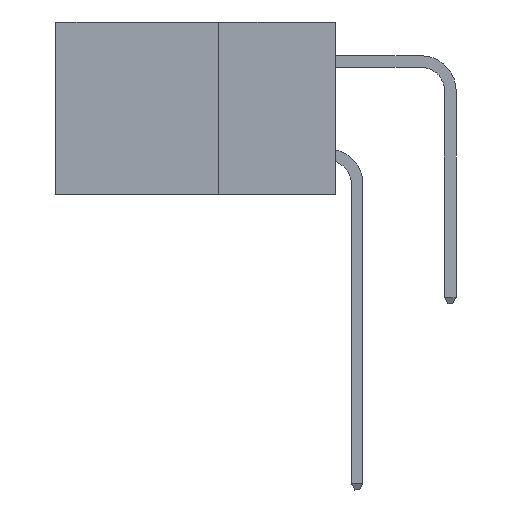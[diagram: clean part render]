
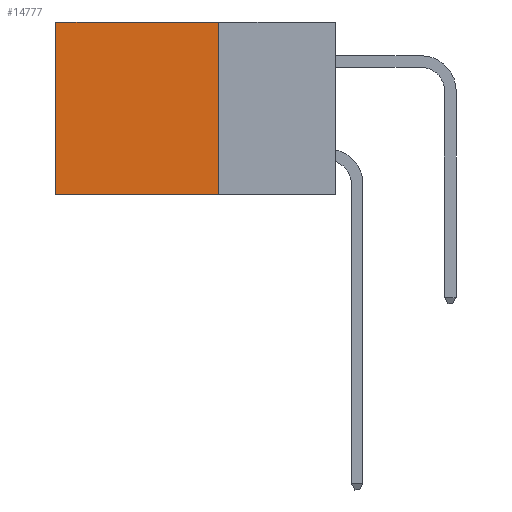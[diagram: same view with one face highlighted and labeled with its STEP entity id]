
A CAD part, left-side view. The second image highlights one B-rep face of the part: STEP entity #14777.
In plain terms, the highlighted planar face has unit normal (-1, 0, 0).
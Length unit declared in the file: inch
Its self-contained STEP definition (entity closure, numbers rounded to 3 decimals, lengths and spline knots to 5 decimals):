
#572 = EDGE_LOOP ( 'NONE', ( #13599, #17143, #7710, #5139 ) ) ;
#2084 = VECTOR ( 'NONE', #3341, 39.37008 ) ;
#3341 = DIRECTION ( 'NONE',  ( 0., 0., -1. ) ) ;
#3626 = CARTESIAN_POINT ( 'NONE',  ( 0.2875, 0.25, 0. ) ) ;
#3727 = CARTESIAN_POINT ( 'NONE',  ( 0.2875, 0.6, 0. ) ) ;
#4775 = CARTESIAN_POINT ( 'NONE',  ( 0.2875, 0.6, 0. ) ) ;
#4936 = AXIS2_PLACEMENT_3D ( 'NONE', #16411, #18067, #8132 ) ;
#5107 = LINE ( 'NONE', #3727, #8947 ) ;
#5139 = ORIENTED_EDGE ( 'NONE', *, *, #15364, .T. ) ;
#5834 = EDGE_CURVE ( 'NONE', #14093, #7634, #5107, .T. ) ;
#5984 = CARTESIAN_POINT ( 'NONE',  ( 0.2875, 0.25, -0.37 ) ) ;
#6484 = PLANE ( 'NONE',  #4936 ) ;
#7013 = FACE_OUTER_BOUND ( 'NONE', #572, .T. ) ;
#7097 = LINE ( 'NONE', #19820, #15421 ) ;
#7258 = CARTESIAN_POINT ( 'NONE',  ( 0.2875, 0.6, -0.37 ) ) ;
#7440 = EDGE_CURVE ( 'NONE', #9096, #7634, #7097, .T. ) ;
#7634 = VERTEX_POINT ( 'NONE', #7258 ) ;
#7710 = ORIENTED_EDGE ( 'NONE', *, *, #8698, .F. ) ;
#7893 = CARTESIAN_POINT ( 'NONE',  ( 0.2875, 0.25, 0. ) ) ;
#8132 = DIRECTION ( 'NONE',  ( 0., 0., -1. ) ) ;
#8698 = EDGE_CURVE ( 'NONE', #18494, #9096, #19264, .T. ) ;
#8947 = VECTOR ( 'NONE', #17013, 39.37008 ) ;
#9096 = VERTEX_POINT ( 'NONE', #5984 ) ;
#9535 = DIRECTION ( 'NONE',  ( 0., 1., 0. ) ) ;
#12711 = VECTOR ( 'NONE', #9535, 39.37008 ) ;
#13599 = ORIENTED_EDGE ( 'NONE', *, *, #5834, .T. ) ;
#14093 = VERTEX_POINT ( 'NONE', #4775 ) ;
#14777 = ADVANCED_FACE ( 'NONE', ( #7013 ), #6484, .F. ) ;
#14969 = CARTESIAN_POINT ( 'NONE',  ( 0.2875, 0.25, 0. ) ) ;
#15364 = EDGE_CURVE ( 'NONE', #18494, #14093, #17624, .T. ) ;
#15421 = VECTOR ( 'NONE', #21492, 39.37008 ) ;
#16411 = CARTESIAN_POINT ( 'NONE',  ( 0.2875, 0.25, 0. ) ) ;
#17013 = DIRECTION ( 'NONE',  ( 0., 0., -1. ) ) ;
#17143 = ORIENTED_EDGE ( 'NONE', *, *, #7440, .F. ) ;
#17624 = LINE ( 'NONE', #7893, #12711 ) ;
#18067 = DIRECTION ( 'NONE',  ( 1., 0., 0. ) ) ;
#18494 = VERTEX_POINT ( 'NONE', #3626 ) ;
#19264 = LINE ( 'NONE', #14969, #2084 ) ;
#19820 = CARTESIAN_POINT ( 'NONE',  ( 0.2875, 0.25, -0.37 ) ) ;
#21492 = DIRECTION ( 'NONE',  ( 0., 1., 0. ) ) ;
